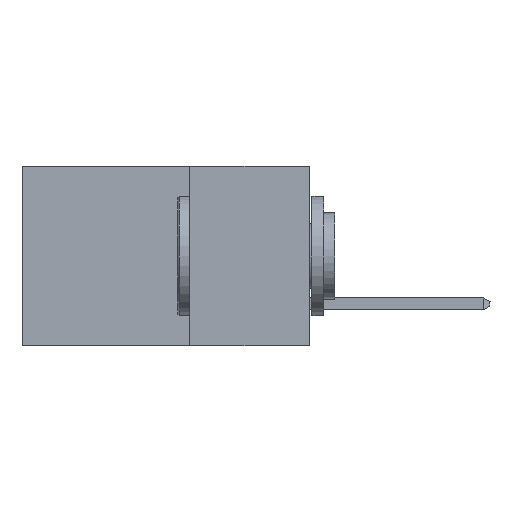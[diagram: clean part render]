
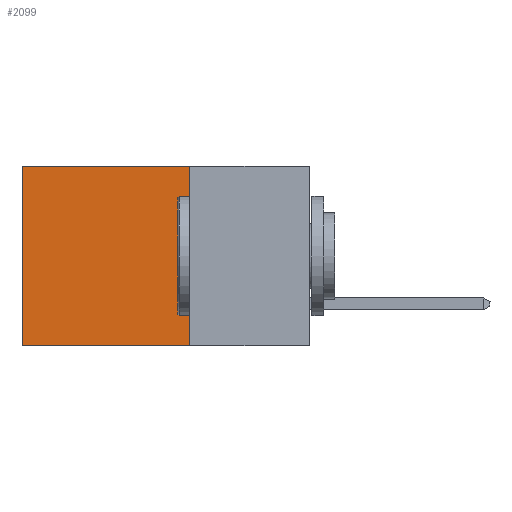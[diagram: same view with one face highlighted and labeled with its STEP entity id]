
A CAD part, left-side view. The second image highlights one B-rep face of the part: STEP entity #2099.
In plain terms, the highlighted planar face has unit normal (-1, 0, 0).
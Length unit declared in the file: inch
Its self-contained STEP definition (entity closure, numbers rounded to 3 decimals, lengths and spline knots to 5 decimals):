
#146 = EDGE_CURVE ( 'NONE', #8826, #4734, #7799, .T. ) ;
#258 = ORIENTED_EDGE ( 'NONE', *, *, #4502, .F. ) ;
#1942 = DIRECTION ( 'NONE',  ( 0., 0., -1. ) ) ;
#2099 = ADVANCED_FACE ( 'NONE', ( #7352 ), #2319, .F. ) ;
#2319 = PLANE ( 'NONE',  #5725 ) ;
#2690 = CARTESIAN_POINT ( 'NONE',  ( 0.2875, 0.6, 0. ) ) ;
#3153 = EDGE_CURVE ( 'NONE', #15114, #3258, #14732, .T. ) ;
#3258 = VERTEX_POINT ( 'NONE', #7936 ) ;
#4138 = VECTOR ( 'NONE', #1942, 39.37008 ) ;
#4260 = DIRECTION ( 'NONE',  ( 0., 1., 0. ) ) ;
#4502 = EDGE_CURVE ( 'NONE', #8826, #15114, #13045, .T. ) ;
#4734 = VERTEX_POINT ( 'NONE', #2690 ) ;
#5435 = VECTOR ( 'NONE', #4260, 39.37008 ) ;
#5665 = DIRECTION ( 'NONE',  ( 0., 0., -1. ) ) ;
#5725 = AXIS2_PLACEMENT_3D ( 'NONE', #9545, #10762, #5809 ) ;
#5809 = DIRECTION ( 'NONE',  ( 0., 0., -1. ) ) ;
#7352 = FACE_OUTER_BOUND ( 'NONE', #15147, .T. ) ;
#7373 = LINE ( 'NONE', #9202, #4138 ) ;
#7799 = LINE ( 'NONE', #11668, #10879 ) ;
#7936 = CARTESIAN_POINT ( 'NONE',  ( 0.2875, 0.6, -0.375 ) ) ;
#8720 = ORIENTED_EDGE ( 'NONE', *, *, #3153, .F. ) ;
#8819 = EDGE_CURVE ( 'NONE', #4734, #3258, #7373, .T. ) ;
#8826 = VERTEX_POINT ( 'NONE', #12564 ) ;
#9202 = CARTESIAN_POINT ( 'NONE',  ( 0.2875, 0.6, -0.375 ) ) ;
#9545 = CARTESIAN_POINT ( 'NONE',  ( 0.2875, 0.25, -0.375 ) ) ;
#9817 = VECTOR ( 'NONE', #5665, 39.37008 ) ;
#10173 = ORIENTED_EDGE ( 'NONE', *, *, #8819, .T. ) ;
#10653 = CARTESIAN_POINT ( 'NONE',  ( 0.2875, 0.25, -0.375 ) ) ;
#10762 = DIRECTION ( 'NONE',  ( 1., 0., 0. ) ) ;
#10879 = VECTOR ( 'NONE', #12866, 39.37008 ) ;
#11668 = CARTESIAN_POINT ( 'NONE',  ( 0.2875, 0.25, 0. ) ) ;
#12564 = CARTESIAN_POINT ( 'NONE',  ( 0.2875, 0.25, 0. ) ) ;
#12866 = DIRECTION ( 'NONE',  ( 0., 1., 0. ) ) ;
#13045 = LINE ( 'NONE', #15397, #9817 ) ;
#14122 = CARTESIAN_POINT ( 'NONE',  ( 0.2875, 0.25, -0.375 ) ) ;
#14727 = ORIENTED_EDGE ( 'NONE', *, *, #146, .T. ) ;
#14732 = LINE ( 'NONE', #14122, #5435 ) ;
#15114 = VERTEX_POINT ( 'NONE', #10653 ) ;
#15147 = EDGE_LOOP ( 'NONE', ( #10173, #8720, #258, #14727 ) ) ;
#15397 = CARTESIAN_POINT ( 'NONE',  ( 0.2875, 0.25, -0.375 ) ) ;
